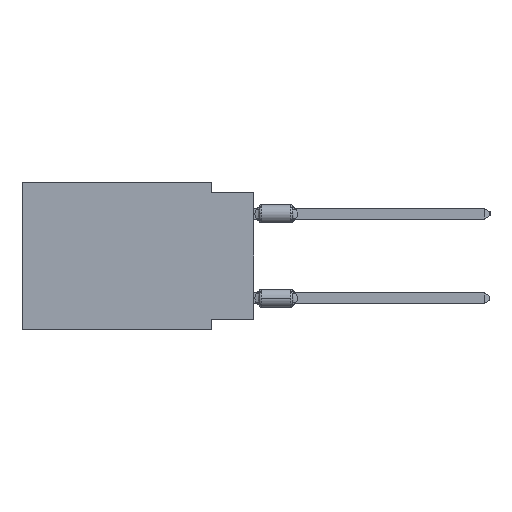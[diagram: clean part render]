
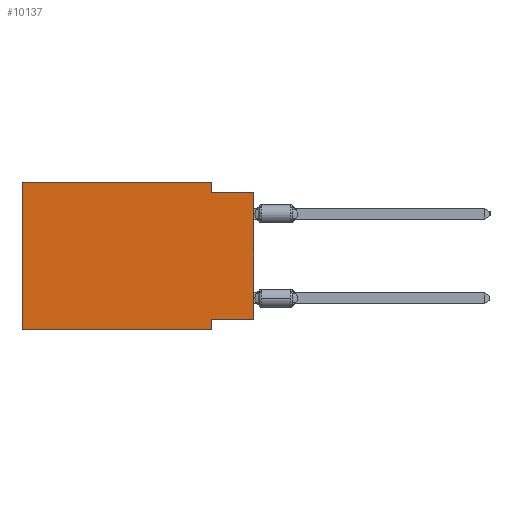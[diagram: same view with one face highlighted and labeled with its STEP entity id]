
A CAD part, left-side view. The second image highlights one B-rep face of the part: STEP entity #10137.
In plain terms, the highlighted planar face has unit normal (-1, 0, 0).
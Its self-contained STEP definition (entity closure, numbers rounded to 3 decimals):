
#800 = LINE ( 'NONE', #19908, #13502 ) ;
#833 = VERTEX_POINT ( 'NONE', #18984 ) ;
#2048 = CARTESIAN_POINT ( 'NONE',  ( 0., 13.97, -8.89 ) ) ;
#2446 = ORIENTED_EDGE ( 'NONE', *, *, #6048, .F. ) ;
#2623 = ORIENTED_EDGE ( 'NONE', *, *, #2813, .F. ) ;
#2813 = EDGE_CURVE ( 'NONE', #14536, #8951, #21004, .T. ) ;
#3501 = CARTESIAN_POINT ( 'NONE',  ( 0., 13.97, 0. ) ) ;
#3916 = CARTESIAN_POINT ( 'NONE',  ( 0., 2.54, -8.89 ) ) ;
#4570 = LINE ( 'NONE', #2048, #7417 ) ;
#4668 = DIRECTION ( 'NONE',  ( 0., -1., 0. ) ) ;
#4739 = EDGE_CURVE ( 'NONE', #14536, #833, #30488, .T. ) ;
#5421 = ORIENTED_EDGE ( 'NONE', *, *, #28611, .F. ) ;
#6048 = EDGE_CURVE ( 'NONE', #7654, #833, #19367, .T. ) ;
#6553 = DIRECTION ( 'NONE',  ( 0., 0., 1. ) ) ;
#7175 = VERTEX_POINT ( 'NONE', #11681 ) ;
#7417 = VECTOR ( 'NONE', #14120, 1000. ) ;
#7457 = ORIENTED_EDGE ( 'NONE', *, *, #4739, .T. ) ;
#7654 = VERTEX_POINT ( 'NONE', #29165 ) ;
#7716 = EDGE_CURVE ( 'NONE', #9214, #7175, #24757, .T. ) ;
#8191 = DIRECTION ( 'NONE',  ( 0., 0., -1. ) ) ;
#8951 = VERTEX_POINT ( 'NONE', #25233 ) ;
#9109 = CARTESIAN_POINT ( 'NONE',  ( 0., 13.97, -8.89 ) ) ;
#9214 = VERTEX_POINT ( 'NONE', #9109 ) ;
#10137 = ADVANCED_FACE ( 'NONE', ( #24950 ), #30123, .F. ) ;
#10401 = VECTOR ( 'NONE', #4668, 1000. ) ;
#10426 = EDGE_CURVE ( 'NONE', #9214, #13150, #4570, .T. ) ;
#11076 = ORIENTED_EDGE ( 'NONE', *, *, #7716, .F. ) ;
#11681 = CARTESIAN_POINT ( 'NONE',  ( 0., 13.97, 0. ) ) ;
#11975 = CARTESIAN_POINT ( 'NONE',  ( 0., 2.54, 0. ) ) ;
#11976 = DIRECTION ( 'NONE',  ( 0., -1., 0. ) ) ;
#13026 = EDGE_CURVE ( 'NONE', #7175, #22591, #16522, .T. ) ;
#13150 = VERTEX_POINT ( 'NONE', #3916 ) ;
#13340 = DIRECTION ( 'NONE',  ( 0., 0., 1. ) ) ;
#13401 = VECTOR ( 'NONE', #6553, 1000. ) ;
#13502 = VECTOR ( 'NONE', #17870, 1000. ) ;
#14120 = DIRECTION ( 'NONE',  ( 0., -1., 0. ) ) ;
#14536 = VERTEX_POINT ( 'NONE', #24569 ) ;
#15348 = VECTOR ( 'NONE', #25557, 1000. ) ;
#16522 = LINE ( 'NONE', #23863, #29463 ) ;
#17261 = VECTOR ( 'NONE', #13340, 1000. ) ;
#17870 = DIRECTION ( 'NONE',  ( 0., 0., -1. ) ) ;
#18736 = EDGE_CURVE ( 'NONE', #22591, #7654, #23855, .T. ) ;
#18984 = CARTESIAN_POINT ( 'NONE',  ( 0., 0., -0.635 ) ) ;
#19054 = CARTESIAN_POINT ( 'NONE',  ( 0., 0., -0.635 ) ) ;
#19367 = LINE ( 'NONE', #19054, #10401 ) ;
#19908 = CARTESIAN_POINT ( 'NONE',  ( 0., 2.54, -8.89 ) ) ;
#21004 = LINE ( 'NONE', #27908, #15348 ) ;
#22127 = ORIENTED_EDGE ( 'NONE', *, *, #10426, .T. ) ;
#22579 = CARTESIAN_POINT ( 'NONE',  ( 0., 2.54, 0. ) ) ;
#22591 = VERTEX_POINT ( 'NONE', #11975 ) ;
#22630 = EDGE_LOOP ( 'NONE', ( #7457, #2446, #25523, #30632, #11076, #22127, #5421, #2623 ) ) ;
#22640 = VECTOR ( 'NONE', #8191, 1000. ) ;
#23855 = LINE ( 'NONE', #22579, #22640 ) ;
#23863 = CARTESIAN_POINT ( 'NONE',  ( 0., 13.97, 0. ) ) ;
#24569 = CARTESIAN_POINT ( 'NONE',  ( 0., 0., -8.255 ) ) ;
#24757 = LINE ( 'NONE', #30237, #17261 ) ;
#24950 = FACE_OUTER_BOUND ( 'NONE', #22630, .T. ) ;
#25233 = CARTESIAN_POINT ( 'NONE',  ( 0., 2.54, -8.255 ) ) ;
#25404 = AXIS2_PLACEMENT_3D ( 'NONE', #3501, #27767, #25421 ) ;
#25421 = DIRECTION ( 'NONE',  ( 0., 0., -1. ) ) ;
#25523 = ORIENTED_EDGE ( 'NONE', *, *, #18736, .F. ) ;
#25557 = DIRECTION ( 'NONE',  ( 0., 1., 0. ) ) ;
#27767 = DIRECTION ( 'NONE',  ( 1., 0., 0. ) ) ;
#27908 = CARTESIAN_POINT ( 'NONE',  ( 0., 0., -8.255 ) ) ;
#27994 = CARTESIAN_POINT ( 'NONE',  ( 0., 0., 0. ) ) ;
#28611 = EDGE_CURVE ( 'NONE', #8951, #13150, #800, .T. ) ;
#29165 = CARTESIAN_POINT ( 'NONE',  ( 0., 2.54, -0.635 ) ) ;
#29463 = VECTOR ( 'NONE', #11976, 1000. ) ;
#30123 = PLANE ( 'NONE',  #25404 ) ;
#30237 = CARTESIAN_POINT ( 'NONE',  ( 0., 13.97, 0. ) ) ;
#30488 = LINE ( 'NONE', #27994, #13401 ) ;
#30632 = ORIENTED_EDGE ( 'NONE', *, *, #13026, .F. ) ;
